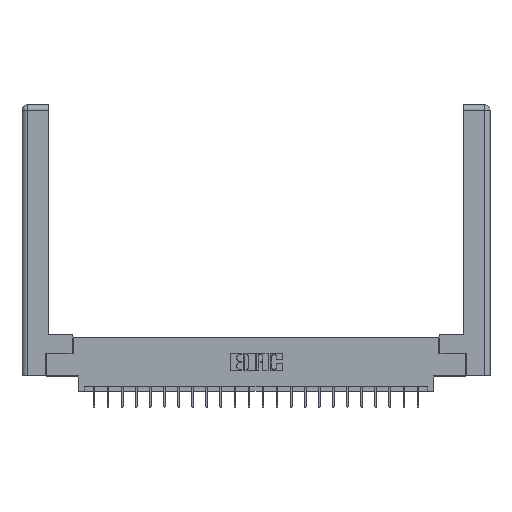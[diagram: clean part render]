
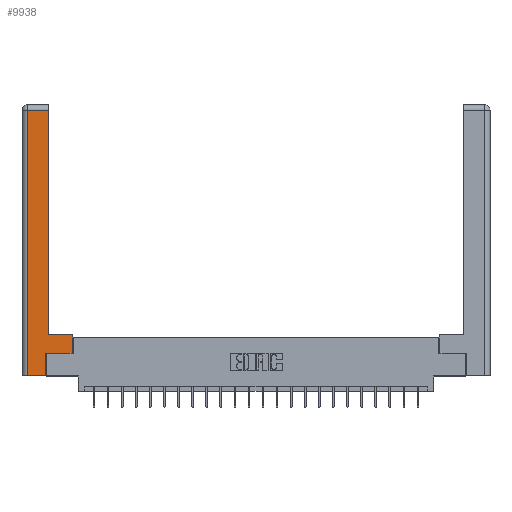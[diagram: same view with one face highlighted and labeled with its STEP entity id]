
A CAD part, top view. The second image highlights one B-rep face of the part: STEP entity #9938.
In plain terms, the highlighted planar face has unit normal (0, 0, 1).
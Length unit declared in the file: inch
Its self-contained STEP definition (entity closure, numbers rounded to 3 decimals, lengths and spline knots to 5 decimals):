
#44 = CARTESIAN_POINT ( 'NONE',  ( 0.565, 0.45, 0. ) ) ;
#162 = CARTESIAN_POINT ( 'NONE',  ( 0.565, 0.45, 0. ) ) ;
#731 = EDGE_CURVE ( 'NONE', #11760, #18514, #17611, .T. ) ;
#1459 = LINE ( 'NONE', #18880, #16069 ) ;
#1530 = LINE ( 'NONE', #7198, #8962 ) ;
#2346 = EDGE_LOOP ( 'NONE', ( #17164, #20886, #19688, #2676, #17912, #13978, #5135, #19107 ) ) ;
#2395 = PLANE ( 'NONE',  #4908 ) ;
#2676 = ORIENTED_EDGE ( 'NONE', *, *, #731, .T. ) ;
#2983 = EDGE_CURVE ( 'NONE', #11489, #12743, #12329, .T. ) ;
#3020 = EDGE_CURVE ( 'NONE', #18514, #11806, #21855, .T. ) ;
#3886 = CARTESIAN_POINT ( 'NONE',  ( 0.265, 0.245, 0. ) ) ;
#4900 = VECTOR ( 'NONE', #23211, 39.37008 ) ;
#4908 = AXIS2_PLACEMENT_3D ( 'NONE', #7898, #17142, #13498 ) ;
#5135 = ORIENTED_EDGE ( 'NONE', *, *, #15628, .T. ) ;
#5165 = VERTEX_POINT ( 'NONE', #162 ) ;
#5288 = CARTESIAN_POINT ( 'NONE',  ( 0.265, 0.245, 0. ) ) ;
#5381 = CARTESIAN_POINT ( 'NONE',  ( 0.0615, 0., 0. ) ) ;
#5550 = DIRECTION ( 'NONE',  ( 0., -1., 0. ) ) ;
#6032 = CARTESIAN_POINT ( 'NONE',  ( 0.265, 0., 0. ) ) ;
#7084 = DIRECTION ( 'NONE',  ( 0., 1., 0. ) ) ;
#7198 = CARTESIAN_POINT ( 'NONE',  ( 0.565, 0.245, 0. ) ) ;
#7370 = VECTOR ( 'NONE', #7084, 39.37008 ) ;
#7788 = CARTESIAN_POINT ( 'NONE',  ( 0.0615, 2.94, 0. ) ) ;
#7858 = DIRECTION ( 'NONE',  ( -1., 0., 0. ) ) ;
#7898 = CARTESIAN_POINT ( 'NONE',  ( 0., 0., 0. ) ) ;
#8962 = VECTOR ( 'NONE', #14399, 39.37008 ) ;
#9743 = VECTOR ( 'NONE', #22059, 39.37008 ) ;
#9938 = ADVANCED_FACE ( 'NONE', ( #16913 ), #2395, .F. ) ;
#11357 = EDGE_CURVE ( 'NONE', #19227, #11489, #12229, .T. ) ;
#11464 = DIRECTION ( 'NONE',  ( 1., 0., 0. ) ) ;
#11489 = VERTEX_POINT ( 'NONE', #18817 ) ;
#11556 = VECTOR ( 'NONE', #11464, 39.37008 ) ;
#11760 = VERTEX_POINT ( 'NONE', #5381 ) ;
#11806 = VERTEX_POINT ( 'NONE', #3886 ) ;
#12229 = LINE ( 'NONE', #19866, #7370 ) ;
#12329 = LINE ( 'NONE', #17994, #4900 ) ;
#12743 = VERTEX_POINT ( 'NONE', #7788 ) ;
#12759 = CARTESIAN_POINT ( 'NONE',  ( 0.0615, 0., 0. ) ) ;
#13498 = DIRECTION ( 'NONE',  ( -1., 0., 0. ) ) ;
#13978 = ORIENTED_EDGE ( 'NONE', *, *, #23051, .T. ) ;
#14347 = LINE ( 'NONE', #44, #9743 ) ;
#14399 = DIRECTION ( 'NONE',  ( 1., 0., 0. ) ) ;
#14455 = CARTESIAN_POINT ( 'NONE',  ( 0.565, 0.245, 0. ) ) ;
#14905 = EDGE_CURVE ( 'NONE', #5165, #19227, #1459, .T. ) ;
#15628 = EDGE_CURVE ( 'NONE', #23754, #5165, #14347, .T. ) ;
#16069 = VECTOR ( 'NONE', #7858, 39.37008 ) ;
#16076 = EDGE_CURVE ( 'NONE', #12743, #11760, #22108, .T. ) ;
#16341 = VECTOR ( 'NONE', #5550, 39.37008 ) ;
#16913 = FACE_OUTER_BOUND ( 'NONE', #2346, .T. ) ;
#17142 = DIRECTION ( 'NONE',  ( 0., 0., -1. ) ) ;
#17164 = ORIENTED_EDGE ( 'NONE', *, *, #11357, .T. ) ;
#17611 = LINE ( 'NONE', #6032, #11556 ) ;
#17912 = ORIENTED_EDGE ( 'NONE', *, *, #3020, .T. ) ;
#17994 = CARTESIAN_POINT ( 'NONE',  ( 0.0615, 2.94, 0. ) ) ;
#18514 = VERTEX_POINT ( 'NONE', #20851 ) ;
#18817 = CARTESIAN_POINT ( 'NONE',  ( 0.295, 2.94, 0. ) ) ;
#18880 = CARTESIAN_POINT ( 'NONE',  ( 0.295, 0.45, 0. ) ) ;
#19107 = ORIENTED_EDGE ( 'NONE', *, *, #14905, .T. ) ;
#19227 = VERTEX_POINT ( 'NONE', #21741 ) ;
#19688 = ORIENTED_EDGE ( 'NONE', *, *, #16076, .T. ) ;
#19866 = CARTESIAN_POINT ( 'NONE',  ( 0.295, 3., 0. ) ) ;
#20851 = CARTESIAN_POINT ( 'NONE',  ( 0.265, 0., 0. ) ) ;
#20886 = ORIENTED_EDGE ( 'NONE', *, *, #2983, .T. ) ;
#21741 = CARTESIAN_POINT ( 'NONE',  ( 0.295, 0.45, 0. ) ) ;
#21855 = LINE ( 'NONE', #5288, #22137 ) ;
#22005 = DIRECTION ( 'NONE',  ( 0., 1., 0. ) ) ;
#22059 = DIRECTION ( 'NONE',  ( 0., 1., 0. ) ) ;
#22108 = LINE ( 'NONE', #12759, #16341 ) ;
#22137 = VECTOR ( 'NONE', #22005, 39.37008 ) ;
#23051 = EDGE_CURVE ( 'NONE', #11806, #23754, #1530, .T. ) ;
#23211 = DIRECTION ( 'NONE',  ( -1., 0., 0. ) ) ;
#23754 = VERTEX_POINT ( 'NONE', #14455 ) ;
